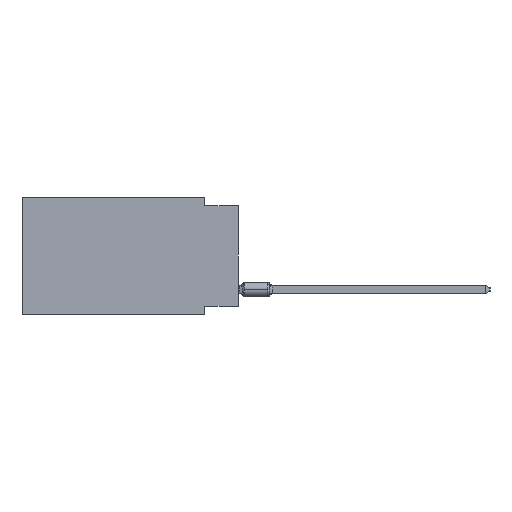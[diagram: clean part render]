
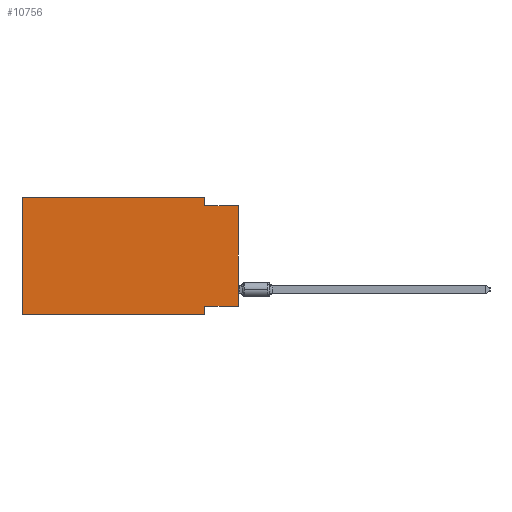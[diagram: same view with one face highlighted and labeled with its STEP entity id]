
A CAD part, left-side view. The second image highlights one B-rep face of the part: STEP entity #10756.
In plain terms, the highlighted planar face has unit normal (-1, 0, 0).
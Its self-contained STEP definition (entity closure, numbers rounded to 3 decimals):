
#747 = LINE ( 'NONE', #11801, #26865 ) ;
#1110 = CARTESIAN_POINT ( 'NONE',  ( 0., 2.54, 0. ) ) ;
#1165 = DIRECTION ( 'NONE',  ( 0., 0., 1. ) ) ;
#1183 = VERTEX_POINT ( 'NONE', #8670 ) ;
#1496 = LINE ( 'NONE', #12029, #21652 ) ;
#2470 = EDGE_CURVE ( 'NONE', #32736, #28981, #7821, .T. ) ;
#3186 = DIRECTION ( 'NONE',  ( 0., -1., 0. ) ) ;
#3321 = CARTESIAN_POINT ( 'NONE',  ( 0., 2.54, 0. ) ) ;
#5749 = EDGE_CURVE ( 'NONE', #5867, #32082, #747, .T. ) ;
#5867 = VERTEX_POINT ( 'NONE', #8607 ) ;
#6065 = CARTESIAN_POINT ( 'NONE',  ( 0., 0., -8.255 ) ) ;
#6819 = CARTESIAN_POINT ( 'NONE',  ( 0., 16.383, 0. ) ) ;
#6839 = ORIENTED_EDGE ( 'NONE', *, *, #2470, .F. ) ;
#7821 = LINE ( 'NONE', #22159, #22092 ) ;
#8251 = CARTESIAN_POINT ( 'NONE',  ( 0., 2.54, -8.89 ) ) ;
#8287 = CARTESIAN_POINT ( 'NONE',  ( 0., 16.383, -8.89 ) ) ;
#8345 = DIRECTION ( 'NONE',  ( 0., 1., 0. ) ) ;
#8381 = VECTOR ( 'NONE', #3186, 1000. ) ;
#8607 = CARTESIAN_POINT ( 'NONE',  ( 0., 2.54, -8.255 ) ) ;
#8621 = LINE ( 'NONE', #29328, #20462 ) ;
#8670 = CARTESIAN_POINT ( 'NONE',  ( 0., 16.383, -8.89 ) ) ;
#10342 = LINE ( 'NONE', #8287, #8381 ) ;
#10756 = ADVANCED_FACE ( 'NONE', ( #22276 ), #19714, .F. ) ;
#10938 = VECTOR ( 'NONE', #8345, 1000. ) ;
#11556 = CARTESIAN_POINT ( 'NONE',  ( 0., 0., -8.255 ) ) ;
#11699 = CARTESIAN_POINT ( 'NONE',  ( 0., 0., -0.635 ) ) ;
#11801 = CARTESIAN_POINT ( 'NONE',  ( 0., 2.54, -8.89 ) ) ;
#11860 = DIRECTION ( 'NONE',  ( 0., -1., 0. ) ) ;
#12029 = CARTESIAN_POINT ( 'NONE',  ( 0., 16.383, 0. ) ) ;
#13721 = ORIENTED_EDGE ( 'NONE', *, *, #23559, .F. ) ;
#14495 = VERTEX_POINT ( 'NONE', #3321 ) ;
#14687 = DIRECTION ( 'NONE',  ( 0., -1., 0. ) ) ;
#14928 = CARTESIAN_POINT ( 'NONE',  ( 0., 0., 0. ) ) ;
#15907 = ORIENTED_EDGE ( 'NONE', *, *, #27314, .F. ) ;
#16324 = LINE ( 'NONE', #11556, #10938 ) ;
#16559 = EDGE_CURVE ( 'NONE', #21944, #5867, #16324, .T. ) ;
#16617 = CARTESIAN_POINT ( 'NONE',  ( 0., 16.383, 0. ) ) ;
#19714 = PLANE ( 'NONE',  #31280 ) ;
#20126 = CARTESIAN_POINT ( 'NONE',  ( 0., 2.54, -0.635 ) ) ;
#20462 = VECTOR ( 'NONE', #29677, 1000. ) ;
#21181 = ORIENTED_EDGE ( 'NONE', *, *, #23151, .F. ) ;
#21652 = VECTOR ( 'NONE', #11860, 1000. ) ;
#21944 = VERTEX_POINT ( 'NONE', #6065 ) ;
#22002 = VECTOR ( 'NONE', #1165, 1000. ) ;
#22092 = VECTOR ( 'NONE', #14687, 1000. ) ;
#22159 = CARTESIAN_POINT ( 'NONE',  ( 0., 0., -0.635 ) ) ;
#22276 = FACE_OUTER_BOUND ( 'NONE', #22294, .T. ) ;
#22294 = EDGE_LOOP ( 'NONE', ( #27567, #6839, #13721, #21181, #15907, #26556, #32483, #25606 ) ) ;
#23137 = VERTEX_POINT ( 'NONE', #16617 ) ;
#23151 = EDGE_CURVE ( 'NONE', #23137, #14495, #1496, .T. ) ;
#23559 = EDGE_CURVE ( 'NONE', #14495, #32736, #32024, .T. ) ;
#25606 = ORIENTED_EDGE ( 'NONE', *, *, #16559, .F. ) ;
#26556 = ORIENTED_EDGE ( 'NONE', *, *, #28347, .T. ) ;
#26573 = DIRECTION ( 'NONE',  ( 0., 0., -1. ) ) ;
#26865 = VECTOR ( 'NONE', #26573, 1000. ) ;
#27314 = EDGE_CURVE ( 'NONE', #1183, #23137, #8621, .T. ) ;
#27547 = DIRECTION ( 'NONE',  ( 0., 0., -1. ) ) ;
#27567 = ORIENTED_EDGE ( 'NONE', *, *, #31510, .T. ) ;
#27706 = DIRECTION ( 'NONE',  ( 1., 0., 0. ) ) ;
#27823 = LINE ( 'NONE', #14928, #22002 ) ;
#28347 = EDGE_CURVE ( 'NONE', #1183, #32082, #10342, .T. ) ;
#28981 = VERTEX_POINT ( 'NONE', #11699 ) ;
#29328 = CARTESIAN_POINT ( 'NONE',  ( 0., 16.383, 0. ) ) ;
#29658 = DIRECTION ( 'NONE',  ( 0., 0., -1. ) ) ;
#29677 = DIRECTION ( 'NONE',  ( 0., 0., 1. ) ) ;
#31280 = AXIS2_PLACEMENT_3D ( 'NONE', #6819, #27706, #27547 ) ;
#31510 = EDGE_CURVE ( 'NONE', #21944, #28981, #27823, .T. ) ;
#31963 = VECTOR ( 'NONE', #29658, 1000. ) ;
#32024 = LINE ( 'NONE', #1110, #31963 ) ;
#32082 = VERTEX_POINT ( 'NONE', #8251 ) ;
#32483 = ORIENTED_EDGE ( 'NONE', *, *, #5749, .F. ) ;
#32736 = VERTEX_POINT ( 'NONE', #20126 ) ;
